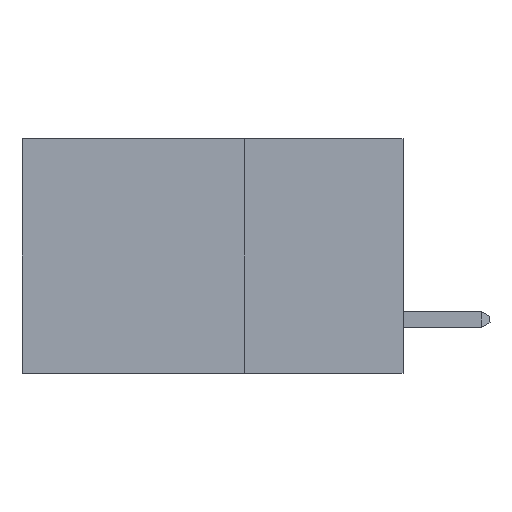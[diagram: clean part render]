
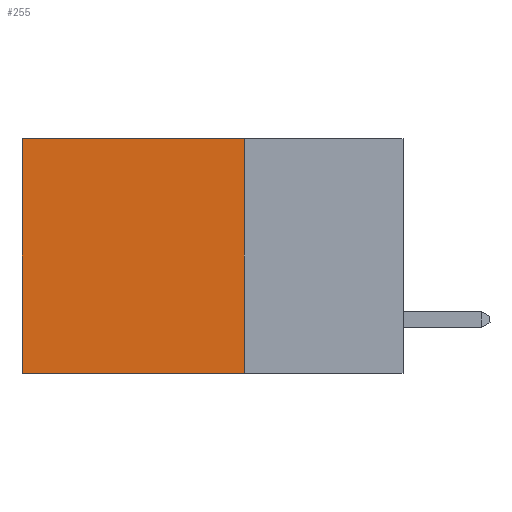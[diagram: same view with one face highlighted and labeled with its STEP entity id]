
A CAD part, left-side view. The second image highlights one B-rep face of the part: STEP entity #255.
In plain terms, the highlighted planar face has unit normal (-1, 0, 0).
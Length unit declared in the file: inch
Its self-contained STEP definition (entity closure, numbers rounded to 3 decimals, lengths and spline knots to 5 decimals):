
#255 = ADVANCED_FACE ( 'NONE', ( #23287 ), #3025, .F. ) ;
#372 = VERTEX_POINT ( 'NONE', #2298 ) ;
#641 = ORIENTED_EDGE ( 'NONE', *, *, #7413, .T. ) ;
#2214 = DIRECTION ( 'NONE',  ( 0., 0., -1. ) ) ;
#2298 = CARTESIAN_POINT ( 'NONE',  ( 0.2875, 0.6, 0. ) ) ;
#2327 = DIRECTION ( 'NONE',  ( 1., 0., 0. ) ) ;
#2385 = VERTEX_POINT ( 'NONE', #16739 ) ;
#2753 = CARTESIAN_POINT ( 'NONE',  ( 0.2875, 0.25, 0. ) ) ;
#3025 = PLANE ( 'NONE',  #21409 ) ;
#3376 = ORIENTED_EDGE ( 'NONE', *, *, #24082, .T. ) ;
#3674 = EDGE_CURVE ( 'NONE', #10249, #6359, #25840, .T. ) ;
#4558 = VECTOR ( 'NONE', #5016, 39.37008 ) ;
#4797 = CARTESIAN_POINT ( 'NONE',  ( 0.2875, 0.6, -0.37 ) ) ;
#5016 = DIRECTION ( 'NONE',  ( 0., 1., 0. ) ) ;
#5552 = EDGE_LOOP ( 'NONE', ( #641, #25542, #6330, #3376 ) ) ;
#6180 = CARTESIAN_POINT ( 'NONE',  ( 0.2875, 0.25, -0.37 ) ) ;
#6330 = ORIENTED_EDGE ( 'NONE', *, *, #24778, .F. ) ;
#6359 = VERTEX_POINT ( 'NONE', #4797 ) ;
#7413 = EDGE_CURVE ( 'NONE', #372, #6359, #18597, .T. ) ;
#8373 = DIRECTION ( 'NONE',  ( 0., 0., -1. ) ) ;
#9009 = VECTOR ( 'NONE', #20287, 39.37008 ) ;
#9651 = DIRECTION ( 'NONE',  ( 0., 1., 0. ) ) ;
#10249 = VERTEX_POINT ( 'NONE', #6180 ) ;
#10997 = CARTESIAN_POINT ( 'NONE',  ( 0.2875, 0.25, 0. ) ) ;
#12357 = CARTESIAN_POINT ( 'NONE',  ( 0.2875, 0.25, -0.37 ) ) ;
#13299 = VECTOR ( 'NONE', #8373, 39.37008 ) ;
#16739 = CARTESIAN_POINT ( 'NONE',  ( 0.2875, 0.25, 0. ) ) ;
#18308 = CARTESIAN_POINT ( 'NONE',  ( 0.2875, 0.25, 0. ) ) ;
#18427 = CARTESIAN_POINT ( 'NONE',  ( 0.2875, 0.6, 0. ) ) ;
#18597 = LINE ( 'NONE', #18427, #13299 ) ;
#19705 = LINE ( 'NONE', #18308, #9009 ) ;
#20287 = DIRECTION ( 'NONE',  ( 0., 0., -1. ) ) ;
#20591 = VECTOR ( 'NONE', #9651, 39.37008 ) ;
#21409 = AXIS2_PLACEMENT_3D ( 'NONE', #2753, #2327, #2214 ) ;
#23287 = FACE_OUTER_BOUND ( 'NONE', #5552, .T. ) ;
#24082 = EDGE_CURVE ( 'NONE', #2385, #372, #25881, .T. ) ;
#24778 = EDGE_CURVE ( 'NONE', #2385, #10249, #19705, .T. ) ;
#25542 = ORIENTED_EDGE ( 'NONE', *, *, #3674, .F. ) ;
#25840 = LINE ( 'NONE', #12357, #20591 ) ;
#25881 = LINE ( 'NONE', #10997, #4558 ) ;
